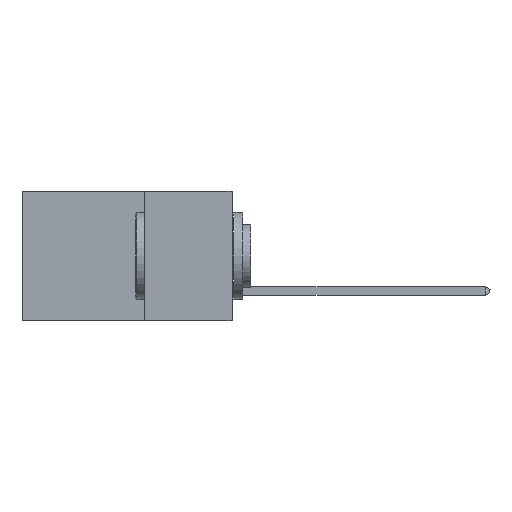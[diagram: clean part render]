
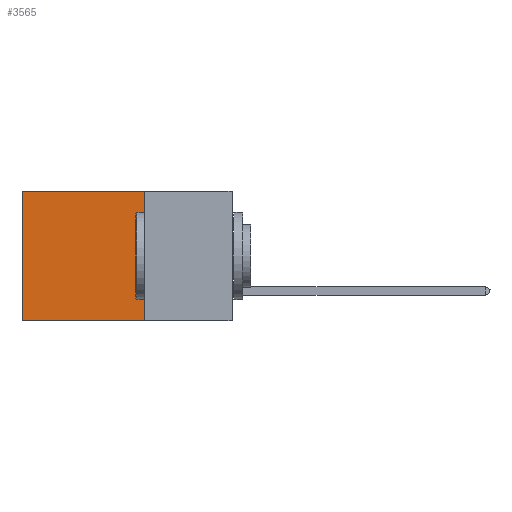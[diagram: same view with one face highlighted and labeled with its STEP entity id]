
A CAD part, left-side view. The second image highlights one B-rep face of the part: STEP entity #3565.
In plain terms, the highlighted planar face has unit normal (-1, 0, 0).
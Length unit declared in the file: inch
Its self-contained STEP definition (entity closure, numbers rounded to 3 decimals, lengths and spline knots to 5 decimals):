
#1038 = ORIENTED_EDGE ( 'NONE', *, *, #42390, .T. ) ;
#2080 = LINE ( 'NONE', #39380, #16514 ) ;
#3433 = EDGE_CURVE ( 'NONE', #30950, #19582, #5137, .T. ) ;
#3565 = ADVANCED_FACE ( 'NONE', ( #14306 ), #32800, .F. ) ;
#3709 = DIRECTION ( 'NONE',  ( 0., 1., 0. ) ) ;
#5137 = LINE ( 'NONE', #39636, #39774 ) ;
#9520 = LINE ( 'NONE', #20097, #22341 ) ;
#9725 = DIRECTION ( 'NONE',  ( 0., 0., -1. ) ) ;
#9866 = CARTESIAN_POINT ( 'NONE',  ( 0.2875, 0.25, 0. ) ) ;
#10294 = ORIENTED_EDGE ( 'NONE', *, *, #3433, .F. ) ;
#12052 = CARTESIAN_POINT ( 'NONE',  ( 0.2875, 0.25, 0. ) ) ;
#14189 = VERTEX_POINT ( 'NONE', #37248 ) ;
#14306 = FACE_OUTER_BOUND ( 'NONE', #37588, .T. ) ;
#14961 = EDGE_CURVE ( 'NONE', #30950, #14189, #2080, .T. ) ;
#16514 = VECTOR ( 'NONE', #26169, 39.37008 ) ;
#19582 = VERTEX_POINT ( 'NONE', #31849 ) ;
#19750 = DIRECTION ( 'NONE',  ( 0., 0., -1. ) ) ;
#20097 = CARTESIAN_POINT ( 'NONE',  ( 0.2875, 0.25, -0.37 ) ) ;
#22341 = VECTOR ( 'NONE', #3709, 39.37008 ) ;
#25387 = CARTESIAN_POINT ( 'NONE',  ( 0.2875, 0.6, 0. ) ) ;
#26169 = DIRECTION ( 'NONE',  ( 0., 1., 0. ) ) ;
#26225 = CARTESIAN_POINT ( 'NONE',  ( 0.2875, 0.6, -0.37 ) ) ;
#28720 = DIRECTION ( 'NONE',  ( 0., 0., -1. ) ) ;
#30950 = VERTEX_POINT ( 'NONE', #12052 ) ;
#31849 = CARTESIAN_POINT ( 'NONE',  ( 0.2875, 0.25, -0.37 ) ) ;
#32784 = ORIENTED_EDGE ( 'NONE', *, *, #36095, .F. ) ;
#32800 = PLANE ( 'NONE',  #35076 ) ;
#34936 = VECTOR ( 'NONE', #28720, 39.37008 ) ;
#35076 = AXIS2_PLACEMENT_3D ( 'NONE', #9866, #39627, #9725 ) ;
#36095 = EDGE_CURVE ( 'NONE', #19582, #37833, #9520, .T. ) ;
#36447 = LINE ( 'NONE', #25387, #34936 ) ;
#36644 = ORIENTED_EDGE ( 'NONE', *, *, #14961, .T. ) ;
#37248 = CARTESIAN_POINT ( 'NONE',  ( 0.2875, 0.6, 0. ) ) ;
#37588 = EDGE_LOOP ( 'NONE', ( #1038, #32784, #10294, #36644 ) ) ;
#37833 = VERTEX_POINT ( 'NONE', #26225 ) ;
#39380 = CARTESIAN_POINT ( 'NONE',  ( 0.2875, 0.25, 0. ) ) ;
#39627 = DIRECTION ( 'NONE',  ( 1., 0., 0. ) ) ;
#39636 = CARTESIAN_POINT ( 'NONE',  ( 0.2875, 0.25, 0. ) ) ;
#39774 = VECTOR ( 'NONE', #19750, 39.37008 ) ;
#42390 = EDGE_CURVE ( 'NONE', #14189, #37833, #36447, .T. ) ;
